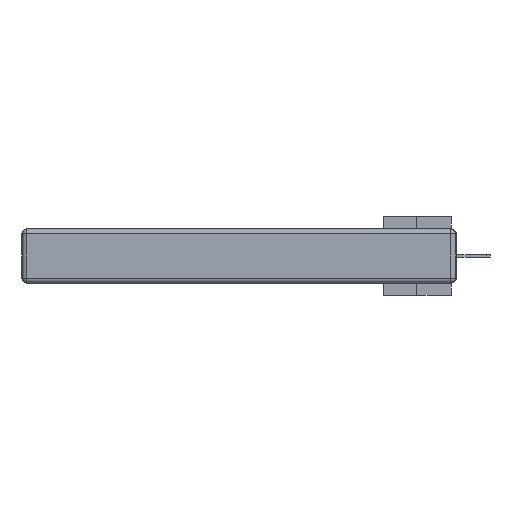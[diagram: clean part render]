
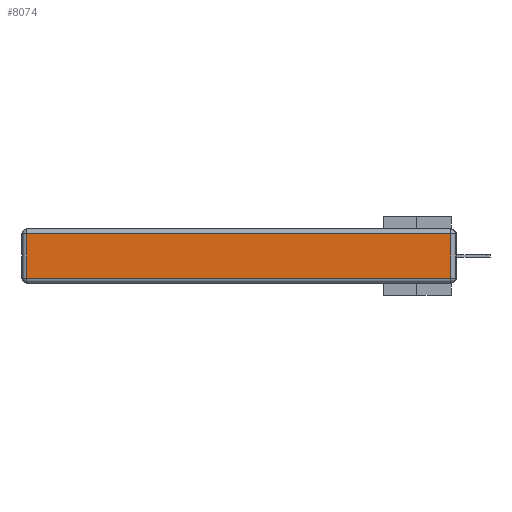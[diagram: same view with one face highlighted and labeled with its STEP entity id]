
A CAD part, left-side view. The second image highlights one B-rep face of the part: STEP entity #8074.
In plain terms, the highlighted planar face has unit normal (-1, 0, 0).
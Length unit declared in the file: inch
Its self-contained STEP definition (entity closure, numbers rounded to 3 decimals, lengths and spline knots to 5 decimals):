
#580 = LINE ( 'NONE', #16188, #21966 ) ;
#1566 = FACE_OUTER_BOUND ( 'NONE', #16711, .T. ) ;
#1647 = DIRECTION ( 'NONE',  ( 0., 0., 1. ) ) ;
#2243 = ORIENTED_EDGE ( 'NONE', *, *, #2363, .T. ) ;
#2363 = EDGE_CURVE ( 'NONE', #6806, #20158, #32694, .T. ) ;
#6116 = ORIENTED_EDGE ( 'NONE', *, *, #13126, .T. ) ;
#6806 = VERTEX_POINT ( 'NONE', #26167 ) ;
#6970 = PLANE ( 'NONE',  #33301 ) ;
#7988 = VERTEX_POINT ( 'NONE', #32050 ) ;
#8074 = ADVANCED_FACE ( 'NONE', ( #1566 ), #6970, .T. ) ;
#9919 = DIRECTION ( 'NONE',  ( 0., 0., 1. ) ) ;
#11852 = VECTOR ( 'NONE', #1647, 39.37008 ) ;
#12040 = CARTESIAN_POINT ( 'NONE',  ( 0., 2.72, -0.313 ) ) ;
#12498 = ORIENTED_EDGE ( 'NONE', *, *, #19849, .T. ) ;
#13126 = EDGE_CURVE ( 'NONE', #20158, #29774, #580, .T. ) ;
#14883 = DIRECTION ( 'NONE',  ( 0., 1., 0. ) ) ;
#15143 = CARTESIAN_POINT ( 'NONE',  ( 0., 2.75, -0.03 ) ) ;
#16188 = CARTESIAN_POINT ( 'NONE',  ( 0., 0., -0.313 ) ) ;
#16711 = EDGE_LOOP ( 'NONE', ( #6116, #12498, #36972, #2243 ) ) ;
#16807 = VECTOR ( 'NONE', #20931, 39.37008 ) ;
#17302 = CARTESIAN_POINT ( 'NONE',  ( 0., 2.72, -0.343 ) ) ;
#17685 = LINE ( 'NONE', #30327, #11852 ) ;
#19849 = EDGE_CURVE ( 'NONE', #29774, #7988, #17685, .T. ) ;
#20158 = VERTEX_POINT ( 'NONE', #12040 ) ;
#20847 = EDGE_CURVE ( 'NONE', #7988, #6806, #29132, .T. ) ;
#20931 = DIRECTION ( 'NONE',  ( 0., 0., -1. ) ) ;
#21933 = DIRECTION ( 'NONE',  ( 0., -1., 0. ) ) ;
#21966 = VECTOR ( 'NONE', #21933, 39.37008 ) ;
#24257 = CARTESIAN_POINT ( 'NONE',  ( 0., 0., -0.343 ) ) ;
#26167 = CARTESIAN_POINT ( 'NONE',  ( 0., 2.72, -0.03 ) ) ;
#26582 = CARTESIAN_POINT ( 'NONE',  ( 0., 0.03, -0.313 ) ) ;
#27062 = DIRECTION ( 'NONE',  ( -1., 0., 0. ) ) ;
#29132 = LINE ( 'NONE', #15143, #36518 ) ;
#29774 = VERTEX_POINT ( 'NONE', #26582 ) ;
#30327 = CARTESIAN_POINT ( 'NONE',  ( 0., 0.03, -0.343 ) ) ;
#32050 = CARTESIAN_POINT ( 'NONE',  ( 0., 0.03, -0.03 ) ) ;
#32694 = LINE ( 'NONE', #17302, #16807 ) ;
#33301 = AXIS2_PLACEMENT_3D ( 'NONE', #24257, #27062, #9919 ) ;
#36518 = VECTOR ( 'NONE', #14883, 39.37008 ) ;
#36972 = ORIENTED_EDGE ( 'NONE', *, *, #20847, .T. ) ;
